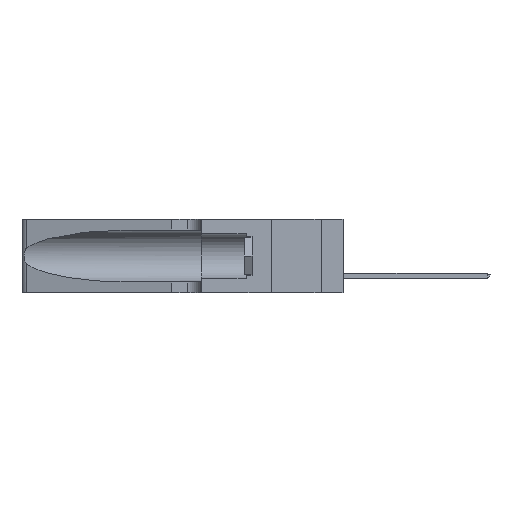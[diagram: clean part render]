
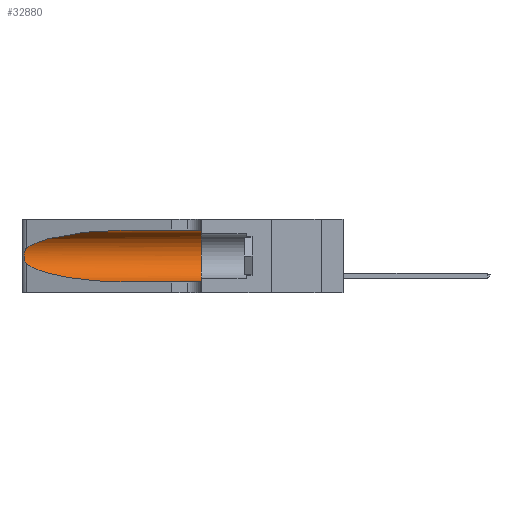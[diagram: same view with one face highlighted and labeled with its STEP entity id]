
A CAD part, left-side view. The second image highlights one B-rep face of the part: STEP entity #32880.
In plain terms, the highlighted cylindrical face has radius 3.308 mm (diameter 6.617 mm), a partial arc.
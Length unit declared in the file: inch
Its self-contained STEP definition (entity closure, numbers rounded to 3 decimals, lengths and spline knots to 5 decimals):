
#83 = AXIS2_PLACEMENT_3D ( 'NONE', #8964, #20558, #2328 ) ;
#745 = CIRCLE ( 'NONE', #4389, 0.13025 ) ;
#2328 = DIRECTION ( 'NONE',  ( 0., 0., -1. ) ) ;
#2461 =( BOUNDED_CURVE ( )  B_SPLINE_CURVE ( 3, ( #26839, #11248, #3530, #16445 ),
 .UNSPECIFIED., .F., .T. ) 
 B_SPLINE_CURVE_WITH_KNOTS ( ( 4, 4 ),
 ( 1.5708, 2.84003 ),
 .UNSPECIFIED. ) 
 CURVE ( )  GEOMETRIC_REPRESENTATION_ITEM ( )  RATIONAL_B_SPLINE_CURVE ( ( 1., 0.87, 0.87, 1. ) ) 
 REPRESENTATION_ITEM ( '' )  );
#3177 = CARTESIAN_POINT ( 'NONE',  ( 0.1305, 0.35, 0.185 ) ) ;
#3213 = CARTESIAN_POINT ( 'NONE',  ( 0.1305, 1.61858, 0.05475 ) ) ;
#3520 = CARTESIAN_POINT ( 'NONE',  ( 0.25854, 1.2359, 0.20912 ) ) ;
#3530 = CARTESIAN_POINT ( 'NONE',  ( 0.2373, 1.15595, 0.28018 ) ) ;
#3861 = VERTEX_POINT ( 'NONE', #26696 ) ;
#4389 = AXIS2_PLACEMENT_3D ( 'NONE', #3177, #21873, #26842 ) ;
#4746 = VECTOR ( 'NONE', #9833, 39.37008 ) ;
#5511 = CARTESIAN_POINT ( 'NONE',  ( 0.25487, 1.22718, 0.14631 ) ) ;
#6442 = CARTESIAN_POINT ( 'NONE',  ( 0.1305, 0.72297, 0.31525 ) ) ;
#7421 = CARTESIAN_POINT ( 'NONE',  ( 0.25487, 1.22718, 0.22369 ) ) ;
#8127 = CARTESIAN_POINT ( 'NONE',  ( 0.25487, 1.22718, 0.22369 ) ) ;
#8471 = CARTESIAN_POINT ( 'NONE',  ( 0.25639, 1.23184, 0.21858 ) ) ;
#8964 = CARTESIAN_POINT ( 'NONE',  ( 0.1305, 1.61858, 0.185 ) ) ;
#9375 = VECTOR ( 'NONE', #19350, 39.37008 ) ;
#9833 = DIRECTION ( 'NONE',  ( 0., -1., 0. ) ) ;
#9873 = EDGE_CURVE ( 'NONE', #13330, #16330, #31766, .T. ) ;
#10426 = CARTESIAN_POINT ( 'NONE',  ( 0.1305, 0.72297, 0.05475 ) ) ;
#10612 = EDGE_CURVE ( 'NONE', #11163, #16330, #745, .T. ) ;
#11163 = VERTEX_POINT ( 'NONE', #19389 ) ;
#11248 = CARTESIAN_POINT ( 'NONE',  ( 0.18966, 0.96281, 0.31525 ) ) ;
#11657 = CYLINDRICAL_SURFACE ( 'NONE', #83, 0.13025 ) ;
#11922 = CARTESIAN_POINT ( 'NONE',  ( 0.25856, 1.23593, 0.16098 ) ) ;
#12248 = ORIENTED_EDGE ( 'NONE', *, *, #28305, .T. ) ;
#12258 = CARTESIAN_POINT ( 'NONE',  ( 0.25639, 1.23186, 0.15144 ) ) ;
#13054 = ORIENTED_EDGE ( 'NONE', *, *, #9873, .T. ) ;
#13191 = EDGE_CURVE ( 'NONE', #30839, #11163, #15749, .T. ) ;
#13263 = FACE_OUTER_BOUND ( 'NONE', #28521, .T. ) ;
#13330 = VERTEX_POINT ( 'NONE', #17424 ) ;
#14412 = CARTESIAN_POINT ( 'NONE',  ( 0.26018, 1.23835, 0.19895 ) ) ;
#14525 = CARTESIAN_POINT ( 'NONE',  ( 0.26017, 1.23833, 0.17102 ) ) ;
#15749 = LINE ( 'NONE', #19618, #4746 ) ;
#16106 = VERTEX_POINT ( 'NONE', #8127 ) ;
#16212 = CARTESIAN_POINT ( 'NONE',  ( 0.25555, 1.22994, 0.2215 ) ) ;
#16330 = VERTEX_POINT ( 'NONE', #25917 ) ;
#16445 = CARTESIAN_POINT ( 'NONE',  ( 0.25487, 1.22718, 0.22369 ) ) ;
#16496 = EDGE_CURVE ( 'NONE', #16106, #3861, #22340, .T. ) ;
#17424 = CARTESIAN_POINT ( 'NONE',  ( 0.1305, 0.72297, 0.05475 ) ) ;
#17466 = CARTESIAN_POINT ( 'NONE',  ( 0.25555, 1.22993, 0.14849 ) ) ;
#18692 =( BOUNDED_CURVE ( )  B_SPLINE_CURVE ( 3, ( #5511, #23769, #20807, #10426 ),
 .UNSPECIFIED., .F., .F. ) 
 B_SPLINE_CURVE_WITH_KNOTS ( ( 4, 4 ),
 ( 3.44316, 4.71239 ),
 .UNSPECIFIED. ) 
 CURVE ( )  GEOMETRIC_REPRESENTATION_ITEM ( )  RATIONAL_B_SPLINE_CURVE ( ( 1., 0.87, 0.87, 1. ) ) 
 REPRESENTATION_ITEM ( '' )  );
#19350 = DIRECTION ( 'NONE',  ( 0., -1., 0. ) ) ;
#19389 = CARTESIAN_POINT ( 'NONE',  ( 0.1305, 0.35, 0.31525 ) ) ;
#19618 = CARTESIAN_POINT ( 'NONE',  ( 0.1305, 1.61858, 0.31525 ) ) ;
#20558 = DIRECTION ( 'NONE',  ( 0., -1., 0. ) ) ;
#20807 = CARTESIAN_POINT ( 'NONE',  ( 0.18966, 0.96281, 0.05475 ) ) ;
#21863 = CARTESIAN_POINT ( 'NONE',  ( 0.25789, 1.23486, 0.15765 ) ) ;
#21873 = DIRECTION ( 'NONE',  ( 0., 1., 0. ) ) ;
#22340 = B_SPLINE_CURVE_WITH_KNOTS ( 'NONE', 3,
 ( #7421, #16212, #8471, #29336, #3520, #14412, #24582, #24916, #14525, #11922, #21863, #12258, #17466, #22744 ),
 .UNSPECIFIED., .F., .F.,
 ( 4, 2, 2, 2, 2, 2, 4 ),
 ( 0., 0.00027, 0.00053, 0.00107, 0.0016, 0.00187, 0.00214 ),
 .UNSPECIFIED. ) ;
#22744 = CARTESIAN_POINT ( 'NONE',  ( 0.25487, 1.22718, 0.14631 ) ) ;
#23622 = ORIENTED_EDGE ( 'NONE', *, *, #16496, .T. ) ;
#23769 = CARTESIAN_POINT ( 'NONE',  ( 0.2373, 1.15595, 0.08982 ) ) ;
#24582 = CARTESIAN_POINT ( 'NONE',  ( 0.26075, 1.23896, 0.19203 ) ) ;
#24916 = CARTESIAN_POINT ( 'NONE',  ( 0.26075, 1.23896, 0.178 ) ) ;
#25319 = ORIENTED_EDGE ( 'NONE', *, *, #31232, .T. ) ;
#25341 = ORIENTED_EDGE ( 'NONE', *, *, #13191, .F. ) ;
#25917 = CARTESIAN_POINT ( 'NONE',  ( 0.1305, 0.35, 0.05475 ) ) ;
#26696 = CARTESIAN_POINT ( 'NONE',  ( 0.25487, 1.22718, 0.14631 ) ) ;
#26839 = CARTESIAN_POINT ( 'NONE',  ( 0.1305, 0.72297, 0.31525 ) ) ;
#26842 = DIRECTION ( 'NONE',  ( 0., 0., 1. ) ) ;
#28301 = ORIENTED_EDGE ( 'NONE', *, *, #10612, .F. ) ;
#28305 = EDGE_CURVE ( 'NONE', #30839, #16106, #2461, .T. ) ;
#28521 = EDGE_LOOP ( 'NONE', ( #12248, #23622, #25319, #13054, #28301, #25341 ) ) ;
#29336 = CARTESIAN_POINT ( 'NONE',  ( 0.25787, 1.23484, 0.2124 ) ) ;
#30839 = VERTEX_POINT ( 'NONE', #6442 ) ;
#31232 = EDGE_CURVE ( 'NONE', #3861, #13330, #18692, .T. ) ;
#31766 = LINE ( 'NONE', #3213, #9375 ) ;
#32880 = ADVANCED_FACE ( 'NONE', ( #13263 ), #11657, .F. ) ;
